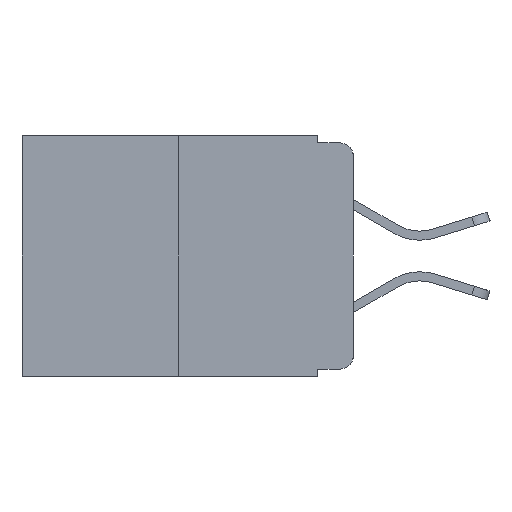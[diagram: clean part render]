
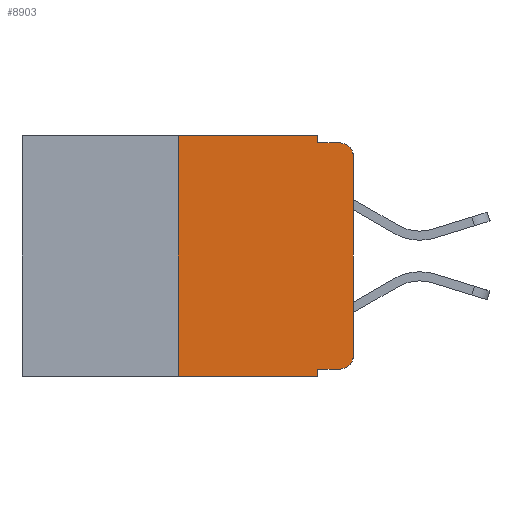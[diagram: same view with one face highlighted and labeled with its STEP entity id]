
A CAD part, left-side view. The second image highlights one B-rep face of the part: STEP entity #8903.
In plain terms, the highlighted planar face has unit normal (-1, 0, 0).
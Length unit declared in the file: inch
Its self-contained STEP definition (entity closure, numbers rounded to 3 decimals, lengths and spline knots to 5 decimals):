
#4 = CARTESIAN_POINT ( 'NONE',  ( 0., 0.02, -0.03 ) ) ;
#140 = LINE ( 'NONE', #4980, #3818 ) ;
#423 = ORIENTED_EDGE ( 'NONE', *, *, #7435, .F. ) ;
#453 = LINE ( 'NONE', #9533, #1759 ) ;
#510 = ORIENTED_EDGE ( 'NONE', *, *, #6704, .F. ) ;
#1244 = VERTEX_POINT ( 'NONE', #7422 ) ;
#1265 = CIRCLE ( 'NONE', #2327, 0.02 ) ;
#1490 = LINE ( 'NONE', #10491, #1931 ) ;
#1659 = DIRECTION ( 'NONE',  ( 0., -1., 0. ) ) ;
#1707 = EDGE_CURVE ( 'NONE', #9888, #4118, #4871, .T. ) ;
#1759 = VECTOR ( 'NONE', #6319, 39.37008 ) ;
#1808 = EDGE_CURVE ( 'NONE', #6138, #1893, #5844, .T. ) ;
#1813 = ORIENTED_EDGE ( 'NONE', *, *, #1707, .T. ) ;
#1823 = CARTESIAN_POINT ( 'NONE',  ( 0., 0.473, 0. ) ) ;
#1893 = VERTEX_POINT ( 'NONE', #9481 ) ;
#1931 = VECTOR ( 'NONE', #9684, 39.37008 ) ;
#2120 = VERTEX_POINT ( 'NONE', #7929 ) ;
#2128 = DIRECTION ( 'NONE',  ( 0., 0., -1. ) ) ;
#2259 = EDGE_CURVE ( 'NONE', #1244, #9561, #8516, .T. ) ;
#2327 = AXIS2_PLACEMENT_3D ( 'NONE', #4, #5812, #3252 ) ;
#2405 = ORIENTED_EDGE ( 'NONE', *, *, #9430, .T. ) ;
#2583 = CARTESIAN_POINT ( 'NONE',  ( 0., 0.473, -0.343 ) ) ;
#2690 = CARTESIAN_POINT ( 'NONE',  ( 0., 0.051, -0.01 ) ) ;
#2727 = CARTESIAN_POINT ( 'NONE',  ( 0., 0.051, 0. ) ) ;
#2730 = ORIENTED_EDGE ( 'NONE', *, *, #9813, .T. ) ;
#2767 = CARTESIAN_POINT ( 'NONE',  ( 0., 0.02, -0.313 ) ) ;
#3129 = VERTEX_POINT ( 'NONE', #2727 ) ;
#3139 = CARTESIAN_POINT ( 'NONE',  ( 0., 0., 0. ) ) ;
#3214 = CARTESIAN_POINT ( 'NONE',  ( 0., 0., -0.313 ) ) ;
#3252 = DIRECTION ( 'NONE',  ( 0., 0., -1. ) ) ;
#3290 = CARTESIAN_POINT ( 'NONE',  ( 0., 0.25, -0.343 ) ) ;
#3516 = CARTESIAN_POINT ( 'NONE',  ( 0., 0.02, -0.333 ) ) ;
#3602 = EDGE_CURVE ( 'NONE', #2120, #1893, #9520, .T. ) ;
#3818 = VECTOR ( 'NONE', #4269, 39.37008 ) ;
#3868 = AXIS2_PLACEMENT_3D ( 'NONE', #2767, #6993, #9350 ) ;
#4051 = CIRCLE ( 'NONE', #3868, 0.02 ) ;
#4118 = VERTEX_POINT ( 'NONE', #8634 ) ;
#4269 = DIRECTION ( 'NONE',  ( 0., 0., 1. ) ) ;
#4764 = DIRECTION ( 'NONE',  ( 0., 0., 1. ) ) ;
#4871 = LINE ( 'NONE', #3139, #8392 ) ;
#4979 = EDGE_LOOP ( 'NONE', ( #1813, #5777, #8890, #6698, #510, #423, #8297, #5052, #2405, #2730 ) ) ;
#4980 = CARTESIAN_POINT ( 'NONE',  ( 0., 0.25, 0. ) ) ;
#5052 = ORIENTED_EDGE ( 'NONE', *, *, #3602, .F. ) ;
#5651 = EDGE_CURVE ( 'NONE', #4118, #9561, #1265, .T. ) ;
#5777 = ORIENTED_EDGE ( 'NONE', *, *, #5651, .T. ) ;
#5812 = DIRECTION ( 'NONE',  ( -1., 0., 0. ) ) ;
#5844 = LINE ( 'NONE', #2583, #7046 ) ;
#6009 = DIRECTION ( 'NONE',  ( 0., 0., -1. ) ) ;
#6138 = VERTEX_POINT ( 'NONE', #3290 ) ;
#6319 = DIRECTION ( 'NONE',  ( 0., 0., -1. ) ) ;
#6698 = ORIENTED_EDGE ( 'NONE', *, *, #9419, .F. ) ;
#6704 = EDGE_CURVE ( 'NONE', #8616, #3129, #6731, .T. ) ;
#6731 = LINE ( 'NONE', #9992, #7560 ) ;
#6893 = VECTOR ( 'NONE', #2128, 39.37008 ) ;
#6978 = DIRECTION ( 'NONE',  ( 1., 0., 0. ) ) ;
#6993 = DIRECTION ( 'NONE',  ( -1., 0., 0. ) ) ;
#7046 = VECTOR ( 'NONE', #1659, 39.37008 ) ;
#7381 = CARTESIAN_POINT ( 'NONE',  ( 0., 0.02, -0.01 ) ) ;
#7422 = CARTESIAN_POINT ( 'NONE',  ( 0., 0.051, -0.01 ) ) ;
#7435 = EDGE_CURVE ( 'NONE', #6138, #8616, #140, .T. ) ;
#7560 = VECTOR ( 'NONE', #9248, 39.37008 ) ;
#7929 = CARTESIAN_POINT ( 'NONE',  ( 0., 0.051, -0.333 ) ) ;
#8297 = ORIENTED_EDGE ( 'NONE', *, *, #1808, .T. ) ;
#8300 = AXIS2_PLACEMENT_3D ( 'NONE', #1823, #6978, #6009 ) ;
#8392 = VECTOR ( 'NONE', #4764, 39.37008 ) ;
#8516 = LINE ( 'NONE', #2690, #9453 ) ;
#8616 = VERTEX_POINT ( 'NONE', #8820 ) ;
#8634 = CARTESIAN_POINT ( 'NONE',  ( 0., 0., -0.03 ) ) ;
#8820 = CARTESIAN_POINT ( 'NONE',  ( 0., 0.25, 0. ) ) ;
#8890 = ORIENTED_EDGE ( 'NONE', *, *, #2259, .F. ) ;
#8903 = ADVANCED_FACE ( 'NONE', ( #9226 ), #10080, .F. ) ;
#9226 = FACE_OUTER_BOUND ( 'NONE', #4979, .T. ) ;
#9248 = DIRECTION ( 'NONE',  ( 0., -1., 0. ) ) ;
#9350 = DIRECTION ( 'NONE',  ( 0., 0., -1. ) ) ;
#9388 = DIRECTION ( 'NONE',  ( 0., -1., 0. ) ) ;
#9419 = EDGE_CURVE ( 'NONE', #3129, #1244, #453, .T. ) ;
#9430 = EDGE_CURVE ( 'NONE', #2120, #10147, #1490, .T. ) ;
#9453 = VECTOR ( 'NONE', #9388, 39.37008 ) ;
#9481 = CARTESIAN_POINT ( 'NONE',  ( 0., 0.051, -0.343 ) ) ;
#9520 = LINE ( 'NONE', #10319, #6893 ) ;
#9533 = CARTESIAN_POINT ( 'NONE',  ( 0., 0.051, 0. ) ) ;
#9561 = VERTEX_POINT ( 'NONE', #7381 ) ;
#9684 = DIRECTION ( 'NONE',  ( 0., -1., 0. ) ) ;
#9813 = EDGE_CURVE ( 'NONE', #10147, #9888, #4051, .T. ) ;
#9888 = VERTEX_POINT ( 'NONE', #3214 ) ;
#9992 = CARTESIAN_POINT ( 'NONE',  ( 0., 0.473, 0. ) ) ;
#10080 = PLANE ( 'NONE',  #8300 ) ;
#10147 = VERTEX_POINT ( 'NONE', #3516 ) ;
#10319 = CARTESIAN_POINT ( 'NONE',  ( 0., 0.051, 0. ) ) ;
#10491 = CARTESIAN_POINT ( 'NONE',  ( 0., 0.051, -0.333 ) ) ;
